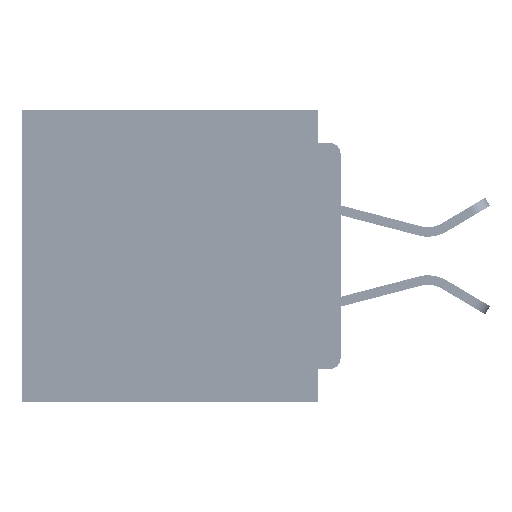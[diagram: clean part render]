
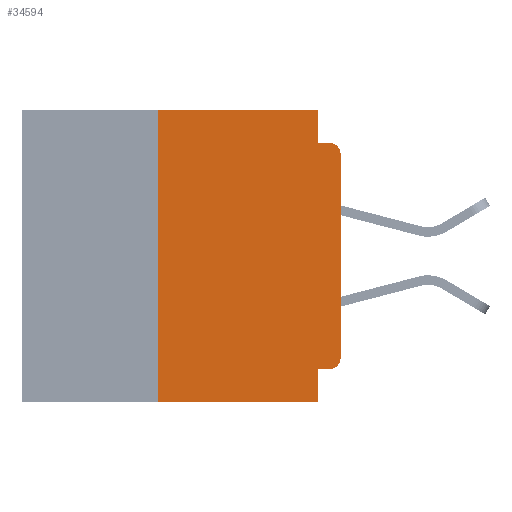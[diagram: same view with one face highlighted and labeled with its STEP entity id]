
A CAD part, left-side view. The second image highlights one B-rep face of the part: STEP entity #34594.
In plain terms, the highlighted planar face has unit normal (-1, 0, 0).
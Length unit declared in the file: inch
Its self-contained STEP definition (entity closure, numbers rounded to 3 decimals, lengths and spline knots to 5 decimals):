
#1078 = CIRCLE ( 'NONE', #34347, 0.015 ) ;
#1121 = EDGE_CURVE ( 'NONE', #2849, #45685, #39367, .T. ) ;
#2849 = VERTEX_POINT ( 'NONE', #58054 ) ;
#4116 = LINE ( 'NONE', #10258, #45965 ) ;
#4689 = CARTESIAN_POINT ( 'NONE',  ( 0., 0.437, 0. ) ) ;
#4879 = CARTESIAN_POINT ( 'NONE',  ( 0., 0., -0.045 ) ) ;
#6626 = VECTOR ( 'NONE', #32127, 39.37008 ) ;
#7715 = DIRECTION ( 'NONE',  ( 0., 0., -1. ) ) ;
#9594 = VERTEX_POINT ( 'NONE', #29860 ) ;
#10258 = CARTESIAN_POINT ( 'NONE',  ( 0., 0., -0.355 ) ) ;
#10723 = DIRECTION ( 'NONE',  ( -1., 0., 0. ) ) ;
#12188 = ORIENTED_EDGE ( 'NONE', *, *, #41865, .F. ) ;
#12470 = CARTESIAN_POINT ( 'NONE',  ( 0., 0., 0. ) ) ;
#13895 = CARTESIAN_POINT ( 'NONE',  ( 0., 0.031, -0.355 ) ) ;
#13913 = VERTEX_POINT ( 'NONE', #48326 ) ;
#15722 = VERTEX_POINT ( 'NONE', #13895 ) ;
#17831 = AXIS2_PLACEMENT_3D ( 'NONE', #29691, #29603, #29110 ) ;
#18029 = ORIENTED_EDGE ( 'NONE', *, *, #63462, .F. ) ;
#18079 = ORIENTED_EDGE ( 'NONE', *, *, #28570, .T. ) ;
#21111 = CARTESIAN_POINT ( 'NONE',  ( 0., 0.015, -0.045 ) ) ;
#21180 = DIRECTION ( 'NONE',  ( 0., -1., 0. ) ) ;
#22585 = ORIENTED_EDGE ( 'NONE', *, *, #32560, .F. ) ;
#23235 = VERTEX_POINT ( 'NONE', #30763 ) ;
#23267 = CARTESIAN_POINT ( 'NONE',  ( 0., 0.031, 0. ) ) ;
#23482 = DIRECTION ( 'NONE',  ( 0., 0., 1. ) ) ;
#23952 = PLANE ( 'NONE',  #61171 ) ;
#25270 = CARTESIAN_POINT ( 'NONE',  ( 0., 0., -0.34 ) ) ;
#26457 = LINE ( 'NONE', #12470, #57162 ) ;
#27545 = CARTESIAN_POINT ( 'NONE',  ( 0., 0.031, -0.4 ) ) ;
#27973 = ORIENTED_EDGE ( 'NONE', *, *, #1121, .T. ) ;
#28570 = EDGE_CURVE ( 'NONE', #57472, #9594, #40652, .T. ) ;
#29110 = DIRECTION ( 'NONE',  ( 0., 0., -1. ) ) ;
#29455 = CARTESIAN_POINT ( 'NONE',  ( 0., 0.437, 0. ) ) ;
#29603 = DIRECTION ( 'NONE',  ( -1., 0., 0. ) ) ;
#29691 = CARTESIAN_POINT ( 'NONE',  ( 0., 0.015, -0.06 ) ) ;
#29860 = CARTESIAN_POINT ( 'NONE',  ( 0., 0.031, -0.4 ) ) ;
#30161 = EDGE_CURVE ( 'NONE', #13913, #59778, #1078, .T. ) ;
#30763 = CARTESIAN_POINT ( 'NONE',  ( 0., 0.25, 0. ) ) ;
#32053 = EDGE_CURVE ( 'NONE', #57472, #23235, #53687, .T. ) ;
#32127 = DIRECTION ( 'NONE',  ( 0., -1., 0. ) ) ;
#32184 = CARTESIAN_POINT ( 'NONE',  ( 0., 0.25, -0.4 ) ) ;
#32560 = EDGE_CURVE ( 'NONE', #37979, #45685, #37403, .T. ) ;
#34347 = AXIS2_PLACEMENT_3D ( 'NONE', #43453, #10723, #48939 ) ;
#34594 = ADVANCED_FACE ( 'NONE', ( #49041 ), #23952, .F. ) ;
#35988 = DIRECTION ( 'NONE',  ( 0., -1., 0. ) ) ;
#37403 = LINE ( 'NONE', #4879, #6626 ) ;
#37979 = VERTEX_POINT ( 'NONE', #70030 ) ;
#37988 = EDGE_CURVE ( 'NONE', #23235, #43022, #54014, .T. ) ;
#39367 = CIRCLE ( 'NONE', #17831, 0.015 ) ;
#39760 = DIRECTION ( 'NONE',  ( 0., 0., -1. ) ) ;
#39970 = ORIENTED_EDGE ( 'NONE', *, *, #51990, .F. ) ;
#40435 = DIRECTION ( 'NONE',  ( 1., 0., 0. ) ) ;
#40652 = LINE ( 'NONE', #68594, #53457 ) ;
#41865 = EDGE_CURVE ( 'NONE', #43022, #37979, #57763, .T. ) ;
#43022 = VERTEX_POINT ( 'NONE', #44147 ) ;
#43453 = CARTESIAN_POINT ( 'NONE',  ( 0., 0.015, -0.34 ) ) ;
#44033 = DIRECTION ( 'NONE',  ( 0., 0., -1. ) ) ;
#44147 = CARTESIAN_POINT ( 'NONE',  ( 0., 0.031, 0. ) ) ;
#44304 = LINE ( 'NONE', #27545, #57060 ) ;
#45685 = VERTEX_POINT ( 'NONE', #21111 ) ;
#45965 = VECTOR ( 'NONE', #48462, 39.37008 ) ;
#46308 = EDGE_CURVE ( 'NONE', #59778, #2849, #26457, .T. ) ;
#48326 = CARTESIAN_POINT ( 'NONE',  ( 0., 0.015, -0.355 ) ) ;
#48462 = DIRECTION ( 'NONE',  ( 0., 1., 0. ) ) ;
#48939 = DIRECTION ( 'NONE',  ( 0., 0., -1. ) ) ;
#49041 = FACE_OUTER_BOUND ( 'NONE', #58347, .T. ) ;
#51892 = CARTESIAN_POINT ( 'NONE',  ( 0., 0.25, -0.4 ) ) ;
#51990 = EDGE_CURVE ( 'NONE', #13913, #15722, #4116, .T. ) ;
#53457 = VECTOR ( 'NONE', #35988, 39.37008 ) ;
#53687 = LINE ( 'NONE', #32184, #68129 ) ;
#54014 = LINE ( 'NONE', #4689, #66726 ) ;
#56878 = ORIENTED_EDGE ( 'NONE', *, *, #30161, .T. ) ;
#57060 = VECTOR ( 'NONE', #44033, 39.37008 ) ;
#57162 = VECTOR ( 'NONE', #23482, 39.37008 ) ;
#57472 = VERTEX_POINT ( 'NONE', #51892 ) ;
#57763 = LINE ( 'NONE', #23267, #70513 ) ;
#58054 = CARTESIAN_POINT ( 'NONE',  ( 0., 0., -0.06 ) ) ;
#58347 = EDGE_LOOP ( 'NONE', ( #66104, #27973, #22585, #12188, #65772, #59916, #18079, #18029, #39970, #56878 ) ) ;
#59348 = DIRECTION ( 'NONE',  ( 0., 0., 1. ) ) ;
#59778 = VERTEX_POINT ( 'NONE', #25270 ) ;
#59916 = ORIENTED_EDGE ( 'NONE', *, *, #32053, .F. ) ;
#61171 = AXIS2_PLACEMENT_3D ( 'NONE', #29455, #40435, #7715 ) ;
#63462 = EDGE_CURVE ( 'NONE', #15722, #9594, #44304, .T. ) ;
#65772 = ORIENTED_EDGE ( 'NONE', *, *, #37988, .F. ) ;
#66104 = ORIENTED_EDGE ( 'NONE', *, *, #46308, .T. ) ;
#66726 = VECTOR ( 'NONE', #21180, 39.37008 ) ;
#68129 = VECTOR ( 'NONE', #59348, 39.37008 ) ;
#68594 = CARTESIAN_POINT ( 'NONE',  ( 0., 0.437, -0.4 ) ) ;
#70030 = CARTESIAN_POINT ( 'NONE',  ( 0., 0.031, -0.045 ) ) ;
#70513 = VECTOR ( 'NONE', #39760, 39.37008 ) ;
